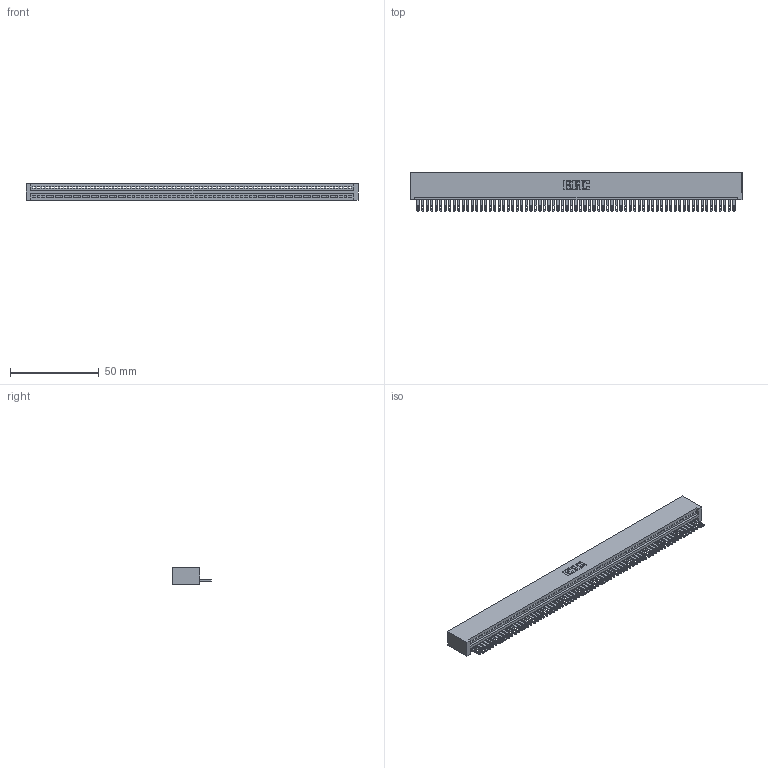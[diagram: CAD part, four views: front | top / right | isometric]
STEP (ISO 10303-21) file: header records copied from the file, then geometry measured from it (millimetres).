
FILE_DESCRIPTION (( 'STEP AP203' ), '1' );
FILE_NAME ('345-071-500-101.STEP', '2019-10-12T19:36:31', ( '' ), ( '' ), 'SwSTEP 2.0', 'SolidWorks 2016', '' );
FILE_SCHEMA (( 'CONFIG_CONTROL_DESIGN' ));
Length unit declared in the file: inch
Products named in the file (3): 345-071-500-101; 345 Part_No Mounting Lugs; 345-292-001_345-293-100
Assembly tree (72 placements, depth 2):
  345-071-500-101
    345 Part_No Mounting Lugs
    345-292-001_345-293-100  x71
Bounding box: 186.94 x 21.51 x 9.4 mm (x, y, z)
Volume: 18622 mm3; surface area: 25490.7 mm2
Topology: 72 solids, 72 shells, 3952 faces, 12245 edges, 8162 vertices
Faces by surface type: plane 2490, cylinder 1462
Entity records: 49185 total; most frequent: ORIENTED_EDGE 8530, CARTESIAN_POINT 8525, DIRECTION 7399, EDGE_CURVE 4265, VECTOR 3853, LINE 3853, VERTEX_POINT 2842, AXIS2_PLACEMENT_3D 1773
